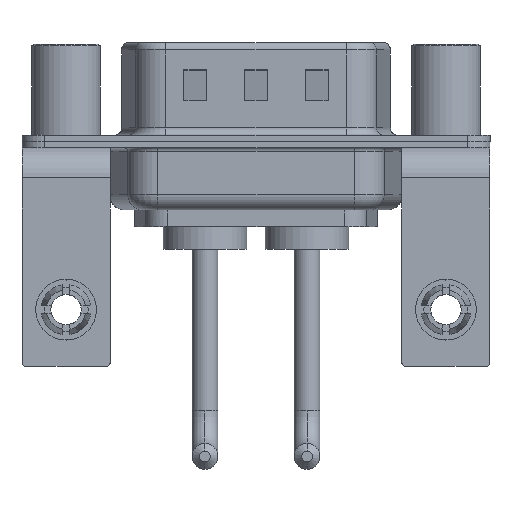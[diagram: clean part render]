
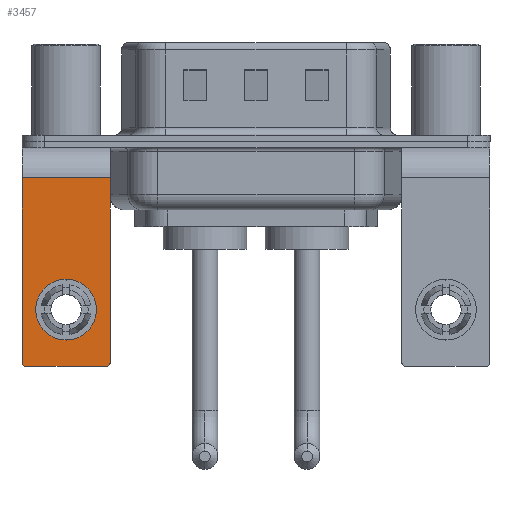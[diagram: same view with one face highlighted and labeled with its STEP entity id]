
A CAD part, front view. The second image highlights one B-rep face of the part: STEP entity #3457.
In plain terms, the highlighted planar face has unit normal (0, -1, 0).
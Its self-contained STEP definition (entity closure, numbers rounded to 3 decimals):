
#18 = FACE_BOUND ( 'NONE', #2520, .T. ) ;
#49 = VECTOR ( 'NONE', #4487, 1000. ) ;
#56 = DIRECTION ( 'NONE',  ( 0., 0., -1. ) ) ;
#98 = CARTESIAN_POINT ( 'NONE',  ( 2.9, -6.25, -2.4 ) ) ;
#144 = DIRECTION ( 'NONE',  ( 0., -1., 0. ) ) ;
#1206 = EDGE_LOOP ( 'NONE', ( #11393, #15001, #15972, #7366, #4541, #4427 ) ) ;
#1505 = EDGE_CURVE ( 'NONE', #6739, #8807, #6969, .T. ) ;
#2520 = EDGE_LOOP ( 'NONE', ( #12158, #17338 ) ) ;
#3072 = VERTEX_POINT ( 'NONE', #16523 ) ;
#3280 = EDGE_CURVE ( 'NONE', #14594, #6739, #11903, .T. ) ;
#3369 = CIRCLE ( 'NONE', #8285, 0.25 ) ;
#3457 = ADVANCED_FACE ( 'NONE', ( #18, #10900 ), #14994, .F. ) ;
#4089 = DIRECTION ( 'NONE',  ( 0., 0., 1. ) ) ;
#4427 = ORIENTED_EDGE ( 'NONE', *, *, #3280, .T. ) ;
#4480 = CARTESIAN_POINT ( 'NONE',  ( -2.65, -6.25, -14.8 ) ) ;
#4487 = DIRECTION ( 'NONE',  ( -1., 0., 0. ) ) ;
#4541 = ORIENTED_EDGE ( 'NONE', *, *, #15931, .F. ) ;
#4588 = VERTEX_POINT ( 'NONE', #13176 ) ;
#4981 = CARTESIAN_POINT ( 'NONE',  ( 2.9, -6.25, -2.4 ) ) ;
#5081 = LINE ( 'NONE', #4981, #10536 ) ;
#5702 = DIRECTION ( 'NONE',  ( 0., 0., 1. ) ) ;
#6461 = EDGE_CURVE ( 'NONE', #8807, #7020, #6534, .T. ) ;
#6534 = CIRCLE ( 'NONE', #10553, 0.25 ) ;
#6739 = VERTEX_POINT ( 'NONE', #6765 ) ;
#6765 = CARTESIAN_POINT ( 'NONE',  ( -2.9, -6.25, -2.4 ) ) ;
#6831 = EDGE_CURVE ( 'NONE', #9229, #8504, #15720, .T. ) ;
#6842 = DIRECTION ( 'NONE',  ( 0., 0., 1. ) ) ;
#6969 = LINE ( 'NONE', #13933, #13796 ) ;
#7020 = VERTEX_POINT ( 'NONE', #4480 ) ;
#7290 = LINE ( 'NONE', #7566, #49 ) ;
#7366 = ORIENTED_EDGE ( 'NONE', *, *, #17527, .T. ) ;
#7428 = CARTESIAN_POINT ( 'NONE',  ( 0., -6.25, -11.07 ) ) ;
#7539 = AXIS2_PLACEMENT_3D ( 'NONE', #98, #17769, #6842 ) ;
#7566 = CARTESIAN_POINT ( 'NONE',  ( 2.9, -6.25, -14.8 ) ) ;
#7952 = AXIS2_PLACEMENT_3D ( 'NONE', #11092, #9738, #13914 ) ;
#8285 = AXIS2_PLACEMENT_3D ( 'NONE', #15295, #11037, #4089 ) ;
#8414 = CARTESIAN_POINT ( 'NONE',  ( 0., -6.25, -9.07 ) ) ;
#8504 = VERTEX_POINT ( 'NONE', #8414 ) ;
#8668 = CARTESIAN_POINT ( 'NONE',  ( -2.65, -6.25, -14.55 ) ) ;
#8807 = VERTEX_POINT ( 'NONE', #16173 ) ;
#8959 = VECTOR ( 'NONE', #10724, 1000. ) ;
#8985 = EDGE_CURVE ( 'NONE', #3072, #7020, #7290, .T. ) ;
#9229 = VERTEX_POINT ( 'NONE', #11993 ) ;
#9738 = DIRECTION ( 'NONE',  ( 0., 1., 0. ) ) ;
#10536 = VECTOR ( 'NONE', #11664, 1000. ) ;
#10553 = AXIS2_PLACEMENT_3D ( 'NONE', #8668, #144, #5702 ) ;
#10724 = DIRECTION ( 'NONE',  ( -1., 0., 0. ) ) ;
#10900 = FACE_OUTER_BOUND ( 'NONE', #1206, .T. ) ;
#11037 = DIRECTION ( 'NONE',  ( 0., -1., 0. ) ) ;
#11092 = CARTESIAN_POINT ( 'NONE',  ( 0., -6.25, -11.07 ) ) ;
#11393 = ORIENTED_EDGE ( 'NONE', *, *, #1505, .T. ) ;
#11403 = DIRECTION ( 'NONE',  ( 0., 0., 1. ) ) ;
#11664 = DIRECTION ( 'NONE',  ( 0., 0., -1. ) ) ;
#11903 = LINE ( 'NONE', #12093, #8959 ) ;
#11993 = CARTESIAN_POINT ( 'NONE',  ( 0., -6.25, -13.07 ) ) ;
#12093 = CARTESIAN_POINT ( 'NONE',  ( 2.9, -6.25, -2.4 ) ) ;
#12158 = ORIENTED_EDGE ( 'NONE', *, *, #6831, .T. ) ;
#12666 = DIRECTION ( 'NONE',  ( 0., 1., 0. ) ) ;
#13176 = CARTESIAN_POINT ( 'NONE',  ( 2.9, -6.25, -14.55 ) ) ;
#13184 = CARTESIAN_POINT ( 'NONE',  ( 2.9, -6.25, -2.4 ) ) ;
#13447 = AXIS2_PLACEMENT_3D ( 'NONE', #7428, #12666, #11403 ) ;
#13796 = VECTOR ( 'NONE', #56, 1000. ) ;
#13914 = DIRECTION ( 'NONE',  ( 0., 0., 1. ) ) ;
#13933 = CARTESIAN_POINT ( 'NONE',  ( -2.9, -6.25, -2.4 ) ) ;
#14594 = VERTEX_POINT ( 'NONE', #13184 ) ;
#14994 = PLANE ( 'NONE',  #7539 ) ;
#15001 = ORIENTED_EDGE ( 'NONE', *, *, #6461, .T. ) ;
#15295 = CARTESIAN_POINT ( 'NONE',  ( 2.65, -6.25, -14.55 ) ) ;
#15720 = CIRCLE ( 'NONE', #7952, 2. ) ;
#15822 = EDGE_CURVE ( 'NONE', #8504, #9229, #17753, .T. ) ;
#15931 = EDGE_CURVE ( 'NONE', #14594, #4588, #5081, .T. ) ;
#15972 = ORIENTED_EDGE ( 'NONE', *, *, #8985, .F. ) ;
#16173 = CARTESIAN_POINT ( 'NONE',  ( -2.9, -6.25, -14.55 ) ) ;
#16523 = CARTESIAN_POINT ( 'NONE',  ( 2.65, -6.25, -14.8 ) ) ;
#17338 = ORIENTED_EDGE ( 'NONE', *, *, #15822, .T. ) ;
#17527 = EDGE_CURVE ( 'NONE', #3072, #4588, #3369, .T. ) ;
#17753 = CIRCLE ( 'NONE', #13447, 2. ) ;
#17769 = DIRECTION ( 'NONE',  ( 0., 1., 0. ) ) ;
